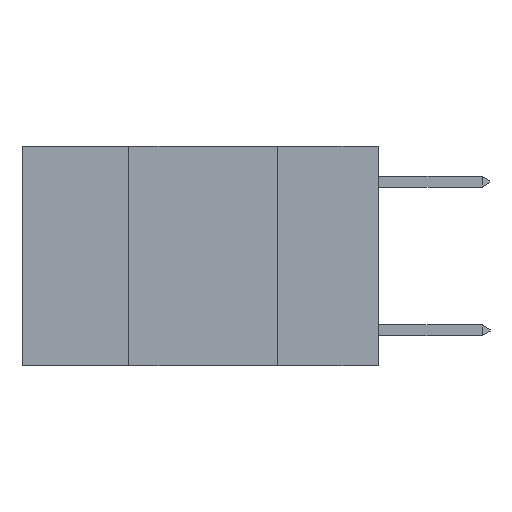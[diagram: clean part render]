
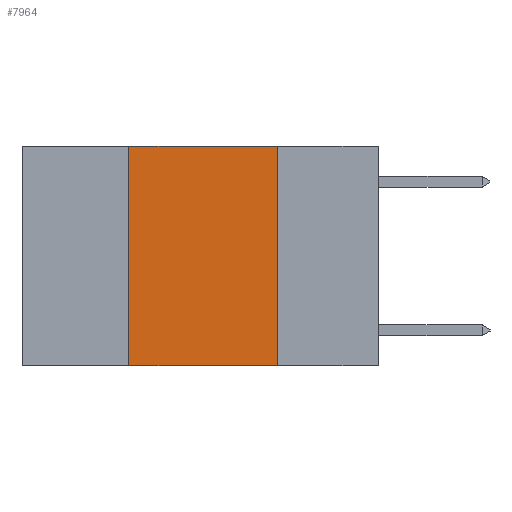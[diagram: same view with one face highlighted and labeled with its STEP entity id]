
A CAD part, left-side view. The second image highlights one B-rep face of the part: STEP entity #7964.
In plain terms, the highlighted planar face has unit normal (-1, 0, 0).
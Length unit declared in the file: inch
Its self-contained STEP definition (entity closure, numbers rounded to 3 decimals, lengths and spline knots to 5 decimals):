
#72 = CARTESIAN_POINT ( 'NONE',  ( 0., 0.6, 0. ) ) ;
#674 = DIRECTION ( 'NONE',  ( 0., 0., -1. ) ) ;
#799 = DIRECTION ( 'NONE',  ( 0., 0., -1. ) ) ;
#1015 = ORIENTED_EDGE ( 'NONE', *, *, #5324, .F. ) ;
#1230 = LINE ( 'NONE', #4147, #4740 ) ;
#1287 = CARTESIAN_POINT ( 'NONE',  ( 0., 0.6, -0.37 ) ) ;
#1786 = LINE ( 'NONE', #5247, #5654 ) ;
#1999 = DIRECTION ( 'NONE',  ( 0., -1., 0. ) ) ;
#2064 = CARTESIAN_POINT ( 'NONE',  ( 0., 0.17, -0.37 ) ) ;
#2838 = EDGE_CURVE ( 'NONE', #5036, #7852, #7898, .T. ) ;
#3051 = ORIENTED_EDGE ( 'NONE', *, *, #5823, .T. ) ;
#3477 = CARTESIAN_POINT ( 'NONE',  ( 0., 0.17, 0. ) ) ;
#4024 = VERTEX_POINT ( 'NONE', #4412 ) ;
#4057 = EDGE_LOOP ( 'NONE', ( #7626, #1015, #4768, #3051 ) ) ;
#4126 = VERTEX_POINT ( 'NONE', #7145 ) ;
#4147 = CARTESIAN_POINT ( 'NONE',  ( 0., 0.6, 0. ) ) ;
#4412 = CARTESIAN_POINT ( 'NONE',  ( 0., 0.42, -0.37 ) ) ;
#4740 = VECTOR ( 'NONE', #5498, 39.37008 ) ;
#4768 = ORIENTED_EDGE ( 'NONE', *, *, #5057, .F. ) ;
#4986 = DIRECTION ( 'NONE',  ( 1., 0., 0. ) ) ;
#5036 = VERTEX_POINT ( 'NONE', #5221 ) ;
#5057 = EDGE_CURVE ( 'NONE', #4024, #4126, #1786, .T. ) ;
#5221 = CARTESIAN_POINT ( 'NONE',  ( 0., 0.17, 0. ) ) ;
#5247 = CARTESIAN_POINT ( 'NONE',  ( 0., 0.42, 0. ) ) ;
#5324 = EDGE_CURVE ( 'NONE', #4126, #5036, #1230, .T. ) ;
#5498 = DIRECTION ( 'NONE',  ( 0., -1., 0. ) ) ;
#5654 = VECTOR ( 'NONE', #5885, 39.37008 ) ;
#5823 = EDGE_CURVE ( 'NONE', #4024, #7852, #8037, .T. ) ;
#5885 = DIRECTION ( 'NONE',  ( 0., 0., 1. ) ) ;
#6114 = VECTOR ( 'NONE', #674, 39.37008 ) ;
#6266 = VECTOR ( 'NONE', #1999, 39.37008 ) ;
#6288 = FACE_OUTER_BOUND ( 'NONE', #4057, .T. ) ;
#7145 = CARTESIAN_POINT ( 'NONE',  ( 0., 0.42, 0. ) ) ;
#7581 = AXIS2_PLACEMENT_3D ( 'NONE', #72, #4986, #799 ) ;
#7626 = ORIENTED_EDGE ( 'NONE', *, *, #2838, .F. ) ;
#7630 = PLANE ( 'NONE',  #7581 ) ;
#7852 = VERTEX_POINT ( 'NONE', #2064 ) ;
#7898 = LINE ( 'NONE', #3477, #6114 ) ;
#7964 = ADVANCED_FACE ( 'NONE', ( #6288 ), #7630, .F. ) ;
#8037 = LINE ( 'NONE', #1287, #6266 ) ;
